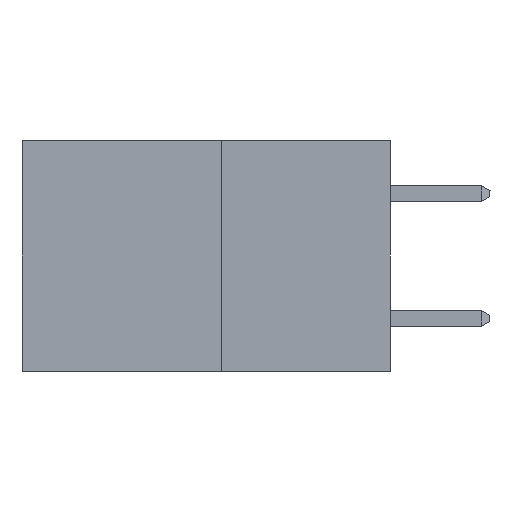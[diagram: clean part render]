
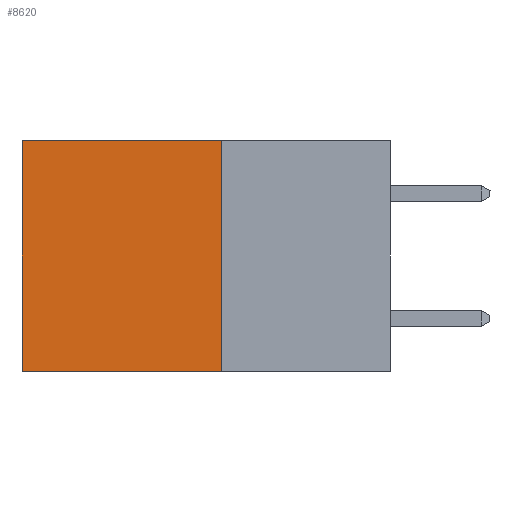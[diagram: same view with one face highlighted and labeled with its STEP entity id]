
A CAD part, left-side view. The second image highlights one B-rep face of the part: STEP entity #8620.
In plain terms, the highlighted planar face has unit normal (-1, 0, 0).
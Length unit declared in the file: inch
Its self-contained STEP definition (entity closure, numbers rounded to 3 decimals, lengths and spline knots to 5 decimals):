
#58 = FACE_OUTER_BOUND ( 'NONE', #4493, .T. ) ;
#1369 = CARTESIAN_POINT ( 'NONE',  ( 0.277, 0.59, -0.37 ) ) ;
#1559 = ORIENTED_EDGE ( 'NONE', *, *, #6522, .F. ) ;
#1574 = DIRECTION ( 'NONE',  ( 0., 1., 0. ) ) ;
#1745 = PLANE ( 'NONE',  #10023 ) ;
#1815 = EDGE_CURVE ( 'NONE', #7539, #2789, #4570, .T. ) ;
#1904 = VECTOR ( 'NONE', #2207, 39.37008 ) ;
#2207 = DIRECTION ( 'NONE',  ( 0., 0., -1. ) ) ;
#2307 = CARTESIAN_POINT ( 'NONE',  ( 0.277, 0.27, 0. ) ) ;
#2789 = VERTEX_POINT ( 'NONE', #6109 ) ;
#3195 = VECTOR ( 'NONE', #9520, 39.37008 ) ;
#4250 = DIRECTION ( 'NONE',  ( 0., 0., -1. ) ) ;
#4364 = VERTEX_POINT ( 'NONE', #5102 ) ;
#4459 = DIRECTION ( 'NONE',  ( 0., 1., 0. ) ) ;
#4493 = EDGE_LOOP ( 'NONE', ( #7924, #10079, #1559, #5987 ) ) ;
#4570 = LINE ( 'NONE', #4621, #8693 ) ;
#4621 = CARTESIAN_POINT ( 'NONE',  ( 0.277, 0.27, -0.37 ) ) ;
#5051 = CARTESIAN_POINT ( 'NONE',  ( 0.277, 0.27, -0.37 ) ) ;
#5102 = CARTESIAN_POINT ( 'NONE',  ( 0.277, 0.59, 0. ) ) ;
#5930 = EDGE_CURVE ( 'NONE', #4364, #2789, #6578, .T. ) ;
#5987 = ORIENTED_EDGE ( 'NONE', *, *, #9702, .T. ) ;
#6042 = VERTEX_POINT ( 'NONE', #2307 ) ;
#6109 = CARTESIAN_POINT ( 'NONE',  ( 0.277, 0.59, -0.37 ) ) ;
#6522 = EDGE_CURVE ( 'NONE', #6042, #7539, #6855, .T. ) ;
#6556 = CARTESIAN_POINT ( 'NONE',  ( 0.277, 0.27, 0. ) ) ;
#6578 = LINE ( 'NONE', #1369, #1904 ) ;
#6855 = LINE ( 'NONE', #8701, #3195 ) ;
#6907 = CARTESIAN_POINT ( 'NONE',  ( 0.277, 0.27, -0.37 ) ) ;
#7539 = VERTEX_POINT ( 'NONE', #6907 ) ;
#7924 = ORIENTED_EDGE ( 'NONE', *, *, #5930, .T. ) ;
#8620 = ADVANCED_FACE ( 'NONE', ( #58 ), #1745, .F. ) ;
#8693 = VECTOR ( 'NONE', #4459, 39.37008 ) ;
#8701 = CARTESIAN_POINT ( 'NONE',  ( 0.277, 0.27, -0.37 ) ) ;
#9180 = DIRECTION ( 'NONE',  ( 1., 0., 0. ) ) ;
#9520 = DIRECTION ( 'NONE',  ( 0., 0., -1. ) ) ;
#9702 = EDGE_CURVE ( 'NONE', #6042, #4364, #9855, .T. ) ;
#9855 = LINE ( 'NONE', #6556, #10114 ) ;
#10023 = AXIS2_PLACEMENT_3D ( 'NONE', #5051, #9180, #4250 ) ;
#10079 = ORIENTED_EDGE ( 'NONE', *, *, #1815, .F. ) ;
#10114 = VECTOR ( 'NONE', #1574, 39.37008 ) ;
